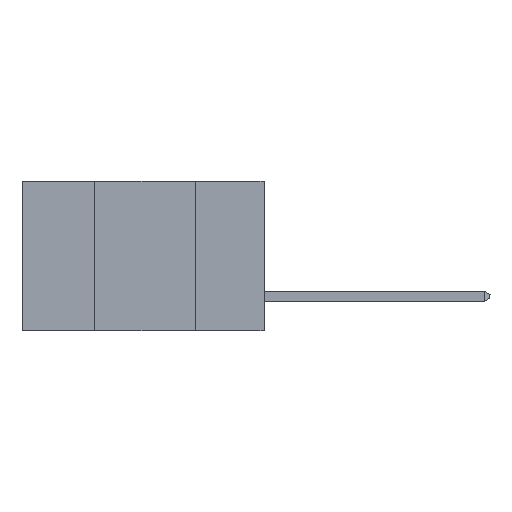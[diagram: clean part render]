
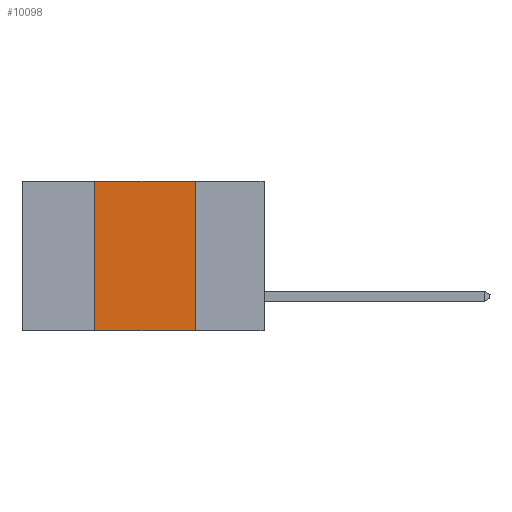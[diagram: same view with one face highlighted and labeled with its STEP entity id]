
A CAD part, left-side view. The second image highlights one B-rep face of the part: STEP entity #10098.
In plain terms, the highlighted planar face has unit normal (-1, 0, 0).
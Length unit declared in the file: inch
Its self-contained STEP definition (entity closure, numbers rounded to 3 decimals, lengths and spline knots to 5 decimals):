
#300 = ORIENTED_EDGE ( 'NONE', *, *, #15430, .F. ) ;
#1557 = EDGE_CURVE ( 'NONE', #2550, #2010, #7332, .T. ) ;
#1919 = VERTEX_POINT ( 'NONE', #12989 ) ;
#2010 = VERTEX_POINT ( 'NONE', #7375 ) ;
#2018 = VECTOR ( 'NONE', #3565, 39.37008 ) ;
#2550 = VERTEX_POINT ( 'NONE', #8102 ) ;
#2960 = EDGE_LOOP ( 'NONE', ( #15843, #300, #13751, #18384 ) ) ;
#3565 = DIRECTION ( 'NONE',  ( 0., -1., 0. ) ) ;
#3576 = DIRECTION ( 'NONE',  ( 0., 0., -1. ) ) ;
#3759 = LINE ( 'NONE', #15549, #2018 ) ;
#3835 = DIRECTION ( 'NONE',  ( 1., 0., 0. ) ) ;
#5511 = LINE ( 'NONE', #16806, #12373 ) ;
#5599 = EDGE_CURVE ( 'NONE', #5963, #2010, #5511, .T. ) ;
#5963 = VERTEX_POINT ( 'NONE', #13518 ) ;
#6302 = EDGE_CURVE ( 'NONE', #2550, #1919, #13679, .T. ) ;
#7228 = DIRECTION ( 'NONE',  ( 0., -1., 0. ) ) ;
#7332 = LINE ( 'NONE', #17634, #11642 ) ;
#7375 = CARTESIAN_POINT ( 'NONE',  ( 0., 0.17, -0.37 ) ) ;
#8102 = CARTESIAN_POINT ( 'NONE',  ( 0., 0.42, -0.37 ) ) ;
#8300 = CARTESIAN_POINT ( 'NONE',  ( 0., 0.6, 0. ) ) ;
#8897 = CARTESIAN_POINT ( 'NONE',  ( 0., 0.42, -0.37 ) ) ;
#10098 = ADVANCED_FACE ( 'NONE', ( #14088 ), #14369, .F. ) ;
#11642 = VECTOR ( 'NONE', #7228, 39.37008 ) ;
#12373 = VECTOR ( 'NONE', #3576, 39.37008 ) ;
#12989 = CARTESIAN_POINT ( 'NONE',  ( 0., 0.42, 0. ) ) ;
#13518 = CARTESIAN_POINT ( 'NONE',  ( 0., 0.17, 0. ) ) ;
#13679 = LINE ( 'NONE', #8897, #17011 ) ;
#13751 = ORIENTED_EDGE ( 'NONE', *, *, #6302, .F. ) ;
#14088 = FACE_OUTER_BOUND ( 'NONE', #2960, .T. ) ;
#14369 = PLANE ( 'NONE',  #14427 ) ;
#14427 = AXIS2_PLACEMENT_3D ( 'NONE', #8300, #3835, #14463 ) ;
#14463 = DIRECTION ( 'NONE',  ( 0., 0., -1. ) ) ;
#15430 = EDGE_CURVE ( 'NONE', #1919, #5963, #3759, .T. ) ;
#15549 = CARTESIAN_POINT ( 'NONE',  ( 0., 0.6, 0. ) ) ;
#15843 = ORIENTED_EDGE ( 'NONE', *, *, #5599, .F. ) ;
#16291 = DIRECTION ( 'NONE',  ( 0., 0., 1. ) ) ;
#16806 = CARTESIAN_POINT ( 'NONE',  ( 0., 0.17, -0.37 ) ) ;
#17011 = VECTOR ( 'NONE', #16291, 39.37008 ) ;
#17634 = CARTESIAN_POINT ( 'NONE',  ( 0., 0.6, -0.37 ) ) ;
#18384 = ORIENTED_EDGE ( 'NONE', *, *, #1557, .T. ) ;
